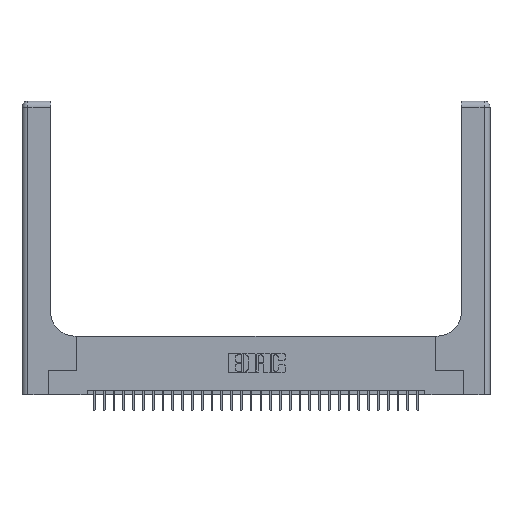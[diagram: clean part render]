
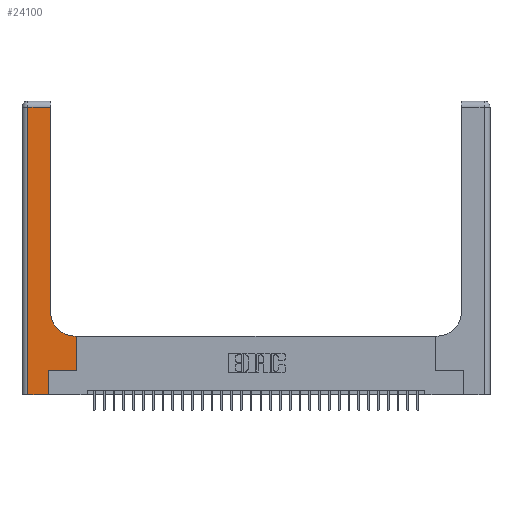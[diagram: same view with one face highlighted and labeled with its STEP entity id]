
A CAD part, top view. The second image highlights one B-rep face of the part: STEP entity #24100.
In plain terms, the highlighted planar face has unit normal (0, 0, 1).
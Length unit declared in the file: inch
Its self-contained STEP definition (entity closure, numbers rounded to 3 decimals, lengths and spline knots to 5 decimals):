
#1131 = DIRECTION ( 'NONE',  ( 0., 0., -1. ) ) ;
#1757 = CARTESIAN_POINT ( 'NONE',  ( 0.269, 0., 0.37 ) ) ;
#1760 = DIRECTION ( 'NONE',  ( 1., 0., 0. ) ) ;
#2196 = LINE ( 'NONE', #9197, #18158 ) ;
#2487 = CARTESIAN_POINT ( 'NONE',  ( 0.5415, 0.6, 0.37 ) ) ;
#2991 = EDGE_CURVE ( 'NONE', #6953, #19893, #12180, .T. ) ;
#3726 = EDGE_CURVE ( 'NONE', #28543, #5066, #13694, .T. ) ;
#3955 = DIRECTION ( 'NONE',  ( 1., 0., 0. ) ) ;
#4677 = AXIS2_PLACEMENT_3D ( 'NONE', #26581, #6327, #31484 ) ;
#4731 = LINE ( 'NONE', #32343, #26621 ) ;
#5066 = VERTEX_POINT ( 'NONE', #2487 ) ;
#5361 = VECTOR ( 'NONE', #3955, 39.37008 ) ;
#5492 = VERTEX_POINT ( 'NONE', #29873 ) ;
#6327 = DIRECTION ( 'NONE',  ( 0., 0., -1. ) ) ;
#6732 = CARTESIAN_POINT ( 'NONE',  ( 0., 2.94, 0.37 ) ) ;
#6812 = DIRECTION ( 'NONE',  ( -1., 0., 0. ) ) ;
#6953 = VERTEX_POINT ( 'NONE', #18989 ) ;
#7415 = LINE ( 'NONE', #32555, #29745 ) ;
#7461 = EDGE_CURVE ( 'NONE', #24037, #28543, #19477, .T. ) ;
#7725 = CARTESIAN_POINT ( 'NONE',  ( 0.269, 0.25, 0.37 ) ) ;
#9197 = CARTESIAN_POINT ( 'NONE',  ( 0.06, 3., 0.37 ) ) ;
#9211 = DIRECTION ( 'NONE',  ( -1., 0., 0. ) ) ;
#10549 = ORIENTED_EDGE ( 'NONE', *, *, #11919, .T. ) ;
#10762 = CARTESIAN_POINT ( 'NONE',  ( 0.5585, 0.25, 0.37 ) ) ;
#11293 = EDGE_LOOP ( 'NONE', ( #12556, #14580, #30349, #26854, #29919, #32481, #13077, #15198, #10549 ) ) ;
#11919 = EDGE_CURVE ( 'NONE', #5066, #31561, #20163, .T. ) ;
#12180 = LINE ( 'NONE', #19214, #5361 ) ;
#12181 = DIRECTION ( 'NONE',  ( -1., 0., 0. ) ) ;
#12556 = ORIENTED_EDGE ( 'NONE', *, *, #25836, .T. ) ;
#12627 = DIRECTION ( 'NONE',  ( 0., 1., 0. ) ) ;
#13077 = ORIENTED_EDGE ( 'NONE', *, *, #7461, .T. ) ;
#13694 = LINE ( 'NONE', #21613, #23622 ) ;
#14322 = DIRECTION ( 'NONE',  ( 0., -1., 0. ) ) ;
#14580 = ORIENTED_EDGE ( 'NONE', *, *, #29702, .T. ) ;
#15198 = ORIENTED_EDGE ( 'NONE', *, *, #3726, .T. ) ;
#15710 = EDGE_CURVE ( 'NONE', #19893, #25360, #4731, .T. ) ;
#17084 = CARTESIAN_POINT ( 'NONE',  ( 0.269, 0.25, 0.37 ) ) ;
#18158 = VECTOR ( 'NONE', #14322, 39.37008 ) ;
#18989 = CARTESIAN_POINT ( 'NONE',  ( 0.06, 0., 0.37 ) ) ;
#19214 = CARTESIAN_POINT ( 'NONE',  ( 0., 0., 0.37 ) ) ;
#19477 = LINE ( 'NONE', #10762, #33001 ) ;
#19893 = VERTEX_POINT ( 'NONE', #1757 ) ;
#20163 = CIRCLE ( 'NONE', #4677, 0.25 ) ;
#20879 = VECTOR ( 'NONE', #12181, 39.37008 ) ;
#21613 = CARTESIAN_POINT ( 'NONE',  ( 0.2915, 0.6, 0.37 ) ) ;
#23582 = VECTOR ( 'NONE', #1760, 39.37008 ) ;
#23622 = VECTOR ( 'NONE', #6812, 39.37008 ) ;
#24037 = VERTEX_POINT ( 'NONE', #31920 ) ;
#24091 = PLANE ( 'NONE',  #24243 ) ;
#24100 = ADVANCED_FACE ( 'NONE', ( #24193 ), #24091, .F. ) ;
#24193 = FACE_OUTER_BOUND ( 'NONE', #11293, .T. ) ;
#24197 = VERTEX_POINT ( 'NONE', #32473 ) ;
#24243 = AXIS2_PLACEMENT_3D ( 'NONE', #29485, #1131, #9211 ) ;
#24557 = CARTESIAN_POINT ( 'NONE',  ( 0.2915, 0.85, 0.37 ) ) ;
#25360 = VERTEX_POINT ( 'NONE', #7725 ) ;
#25641 = EDGE_CURVE ( 'NONE', #5492, #6953, #2196, .T. ) ;
#25836 = EDGE_CURVE ( 'NONE', #31561, #24197, #7415, .T. ) ;
#26581 = CARTESIAN_POINT ( 'NONE',  ( 0.5415, 0.85, 0.37 ) ) ;
#26621 = VECTOR ( 'NONE', #12627, 39.37008 ) ;
#26854 = ORIENTED_EDGE ( 'NONE', *, *, #2991, .T. ) ;
#27424 = EDGE_CURVE ( 'NONE', #25360, #24037, #31603, .T. ) ;
#27432 = DIRECTION ( 'NONE',  ( 0., 1., 0. ) ) ;
#27654 = LINE ( 'NONE', #6732, #20879 ) ;
#28543 = VERTEX_POINT ( 'NONE', #32921 ) ;
#28682 = DIRECTION ( 'NONE',  ( 0., 1., 0. ) ) ;
#29485 = CARTESIAN_POINT ( 'NONE',  ( 0., 3., 0.37 ) ) ;
#29702 = EDGE_CURVE ( 'NONE', #24197, #5492, #27654, .T. ) ;
#29745 = VECTOR ( 'NONE', #27432, 39.37008 ) ;
#29873 = CARTESIAN_POINT ( 'NONE',  ( 0.06, 2.94, 0.37 ) ) ;
#29919 = ORIENTED_EDGE ( 'NONE', *, *, #15710, .T. ) ;
#30349 = ORIENTED_EDGE ( 'NONE', *, *, #25641, .T. ) ;
#31484 = DIRECTION ( 'NONE',  ( 1., 0., 0. ) ) ;
#31561 = VERTEX_POINT ( 'NONE', #24557 ) ;
#31603 = LINE ( 'NONE', #17084, #23582 ) ;
#31920 = CARTESIAN_POINT ( 'NONE',  ( 0.5585, 0.25, 0.37 ) ) ;
#32343 = CARTESIAN_POINT ( 'NONE',  ( 0.269, 0., 0.37 ) ) ;
#32473 = CARTESIAN_POINT ( 'NONE',  ( 0.2915, 2.94, 0.37 ) ) ;
#32481 = ORIENTED_EDGE ( 'NONE', *, *, #27424, .T. ) ;
#32555 = CARTESIAN_POINT ( 'NONE',  ( 0.2915, 3., 0.37 ) ) ;
#32921 = CARTESIAN_POINT ( 'NONE',  ( 0.5585, 0.6, 0.37 ) ) ;
#33001 = VECTOR ( 'NONE', #28682, 39.37008 ) ;
